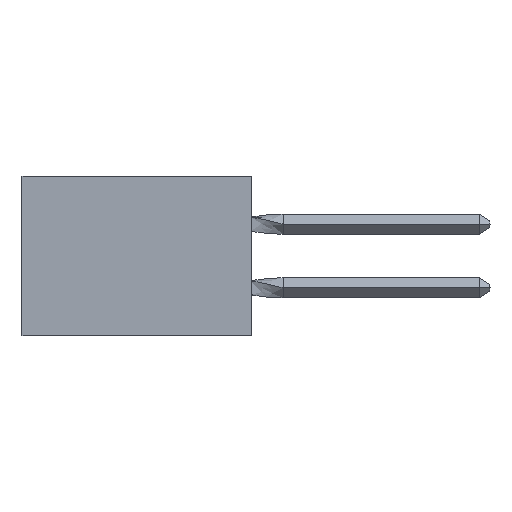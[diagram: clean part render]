
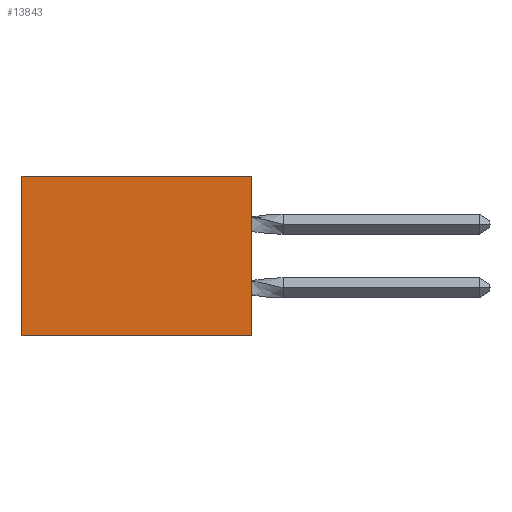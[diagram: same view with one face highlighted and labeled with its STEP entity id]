
A CAD part, left-side view. The second image highlights one B-rep face of the part: STEP entity #13843.
In plain terms, the highlighted planar face has unit normal (-1, 0, 0).
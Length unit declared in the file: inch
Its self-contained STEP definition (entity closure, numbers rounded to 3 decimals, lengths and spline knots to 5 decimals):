
#343 = VECTOR ( 'NONE', #1995, 39.37008 ) ;
#391 = CARTESIAN_POINT ( 'NONE',  ( 0.305, 0., -0.5 ) ) ;
#1469 = CARTESIAN_POINT ( 'NONE',  ( 0.305, 0., -0.5 ) ) ;
#1644 = CARTESIAN_POINT ( 'NONE',  ( 0.305, 0.72, 0. ) ) ;
#1975 = DIRECTION ( 'NONE',  ( 0., 0., -1. ) ) ;
#1995 = DIRECTION ( 'NONE',  ( 0., 0., -1. ) ) ;
#3733 = VERTEX_POINT ( 'NONE', #4724 ) ;
#4441 = ORIENTED_EDGE ( 'NONE', *, *, #20045, .T. ) ;
#4724 = CARTESIAN_POINT ( 'NONE',  ( 0.305, 0.72, -0.5 ) ) ;
#4883 = DIRECTION ( 'NONE',  ( 0., 0., -1. ) ) ;
#5128 = DIRECTION ( 'NONE',  ( 0., 1., 0. ) ) ;
#5859 = EDGE_CURVE ( 'NONE', #6235, #14288, #18821, .T. ) ;
#6014 = ORIENTED_EDGE ( 'NONE', *, *, #12100, .T. ) ;
#6028 = LINE ( 'NONE', #11487, #6767 ) ;
#6235 = VERTEX_POINT ( 'NONE', #8496 ) ;
#6578 = CARTESIAN_POINT ( 'NONE',  ( 0.305, 0., -0.5 ) ) ;
#6767 = VECTOR ( 'NONE', #5128, 39.37008 ) ;
#8496 = CARTESIAN_POINT ( 'NONE',  ( 0.305, 0., 0. ) ) ;
#9439 = VECTOR ( 'NONE', #12488, 39.37008 ) ;
#9566 = AXIS2_PLACEMENT_3D ( 'NONE', #391, #9668, #1975 ) ;
#9668 = DIRECTION ( 'NONE',  ( 1., 0., 0. ) ) ;
#10931 = ORIENTED_EDGE ( 'NONE', *, *, #5859, .F. ) ;
#11461 = VECTOR ( 'NONE', #4883, 39.37008 ) ;
#11487 = CARTESIAN_POINT ( 'NONE',  ( 0.305, 0., 0. ) ) ;
#12100 = EDGE_CURVE ( 'NONE', #6235, #17613, #6028, .T. ) ;
#12488 = DIRECTION ( 'NONE',  ( 0., 1., 0. ) ) ;
#13105 = LINE ( 'NONE', #17320, #9439 ) ;
#13677 = LINE ( 'NONE', #14182, #11461 ) ;
#13843 = ADVANCED_FACE ( 'NONE', ( #18364 ), #16639, .F. ) ;
#14182 = CARTESIAN_POINT ( 'NONE',  ( 0.305, 0.72, -0.5 ) ) ;
#14288 = VERTEX_POINT ( 'NONE', #1469 ) ;
#15543 = EDGE_LOOP ( 'NONE', ( #4441, #15941, #10931, #6014 ) ) ;
#15589 = EDGE_CURVE ( 'NONE', #14288, #3733, #13105, .T. ) ;
#15941 = ORIENTED_EDGE ( 'NONE', *, *, #15589, .F. ) ;
#16639 = PLANE ( 'NONE',  #9566 ) ;
#17320 = CARTESIAN_POINT ( 'NONE',  ( 0.305, 0., -0.5 ) ) ;
#17613 = VERTEX_POINT ( 'NONE', #1644 ) ;
#18364 = FACE_OUTER_BOUND ( 'NONE', #15543, .T. ) ;
#18821 = LINE ( 'NONE', #6578, #343 ) ;
#20045 = EDGE_CURVE ( 'NONE', #17613, #3733, #13677, .T. ) ;
